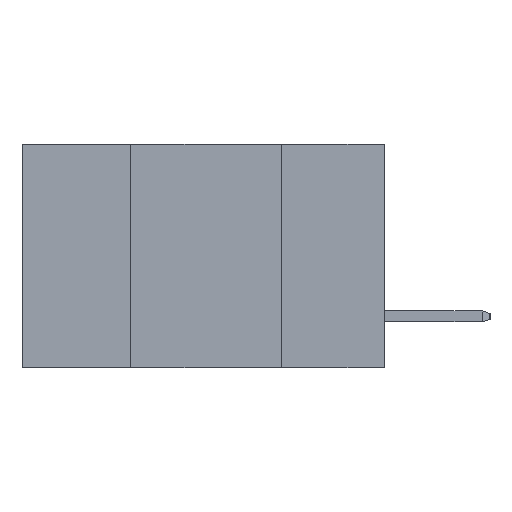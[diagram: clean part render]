
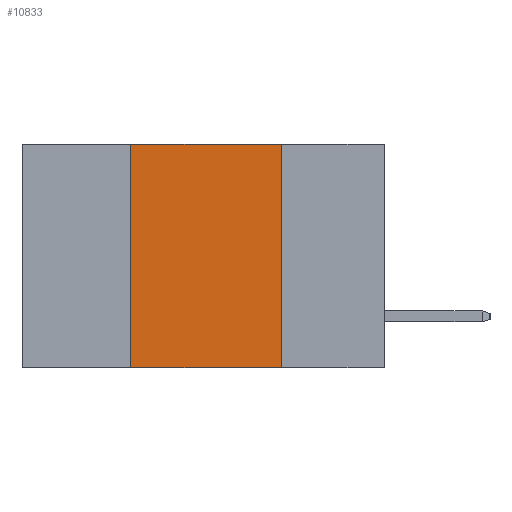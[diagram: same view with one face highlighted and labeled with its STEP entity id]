
A CAD part, left-side view. The second image highlights one B-rep face of the part: STEP entity #10833.
In plain terms, the highlighted planar face has unit normal (-1, 0, 0).
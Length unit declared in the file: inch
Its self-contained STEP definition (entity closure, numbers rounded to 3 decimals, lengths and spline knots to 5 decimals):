
#723 = AXIS2_PLACEMENT_3D ( 'NONE', #4159, #1382, #11069 ) ;
#1382 = DIRECTION ( 'NONE',  ( 1., 0., 0. ) ) ;
#2433 = CARTESIAN_POINT ( 'NONE',  ( 0., 0.42, 0. ) ) ;
#2689 = EDGE_CURVE ( 'NONE', #15861, #13971, #12905, .T. ) ;
#3521 = FACE_OUTER_BOUND ( 'NONE', #11064, .T. ) ;
#4159 = CARTESIAN_POINT ( 'NONE',  ( 0., 0.6, 0. ) ) ;
#4674 = CARTESIAN_POINT ( 'NONE',  ( 0., 0.6, 0. ) ) ;
#5606 = VECTOR ( 'NONE', #10510, 39.37008 ) ;
#6092 = VERTEX_POINT ( 'NONE', #11363 ) ;
#7356 = EDGE_CURVE ( 'NONE', #6092, #15861, #11602, .T. ) ;
#7515 = VERTEX_POINT ( 'NONE', #9911 ) ;
#9163 = VECTOR ( 'NONE', #14476, 39.37008 ) ;
#9591 = LINE ( 'NONE', #13109, #9163 ) ;
#9911 = CARTESIAN_POINT ( 'NONE',  ( 0., 0.17, -0.37 ) ) ;
#10003 = EDGE_CURVE ( 'NONE', #13971, #7515, #10454, .T. ) ;
#10067 = DIRECTION ( 'NONE',  ( 0., 0., -1. ) ) ;
#10138 = CARTESIAN_POINT ( 'NONE',  ( 0., 0.17, -0.37 ) ) ;
#10454 = LINE ( 'NONE', #10138, #14495 ) ;
#10510 = DIRECTION ( 'NONE',  ( 0., -1., 0. ) ) ;
#10592 = ORIENTED_EDGE ( 'NONE', *, *, #7356, .F. ) ;
#10833 = ADVANCED_FACE ( 'NONE', ( #3521 ), #17704, .F. ) ;
#11064 = EDGE_LOOP ( 'NONE', ( #13004, #17325, #10592, #14032 ) ) ;
#11069 = DIRECTION ( 'NONE',  ( 0., 0., -1. ) ) ;
#11309 = DIRECTION ( 'NONE',  ( 0., 0., 1. ) ) ;
#11363 = CARTESIAN_POINT ( 'NONE',  ( 0., 0.42, -0.37 ) ) ;
#11386 = CARTESIAN_POINT ( 'NONE',  ( 0., 0.42, -0.37 ) ) ;
#11602 = LINE ( 'NONE', #11386, #15181 ) ;
#11892 = CARTESIAN_POINT ( 'NONE',  ( 0., 0.17, 0. ) ) ;
#12905 = LINE ( 'NONE', #4674, #5606 ) ;
#13004 = ORIENTED_EDGE ( 'NONE', *, *, #10003, .F. ) ;
#13109 = CARTESIAN_POINT ( 'NONE',  ( 0., 0.6, -0.37 ) ) ;
#13971 = VERTEX_POINT ( 'NONE', #11892 ) ;
#14032 = ORIENTED_EDGE ( 'NONE', *, *, #16286, .T. ) ;
#14476 = DIRECTION ( 'NONE',  ( 0., -1., 0. ) ) ;
#14495 = VECTOR ( 'NONE', #10067, 39.37008 ) ;
#15181 = VECTOR ( 'NONE', #11309, 39.37008 ) ;
#15861 = VERTEX_POINT ( 'NONE', #2433 ) ;
#16286 = EDGE_CURVE ( 'NONE', #6092, #7515, #9591, .T. ) ;
#17325 = ORIENTED_EDGE ( 'NONE', *, *, #2689, .F. ) ;
#17704 = PLANE ( 'NONE',  #723 ) ;
